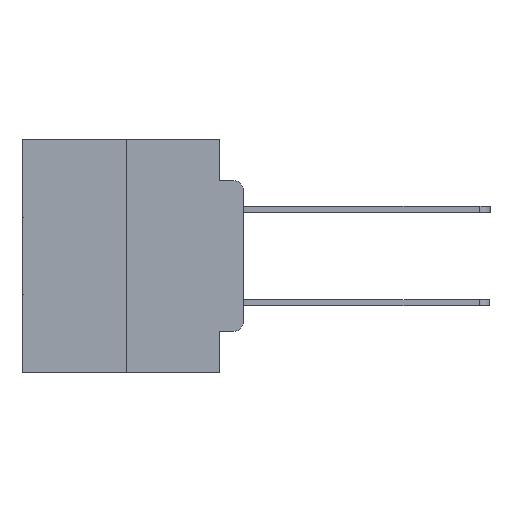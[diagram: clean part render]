
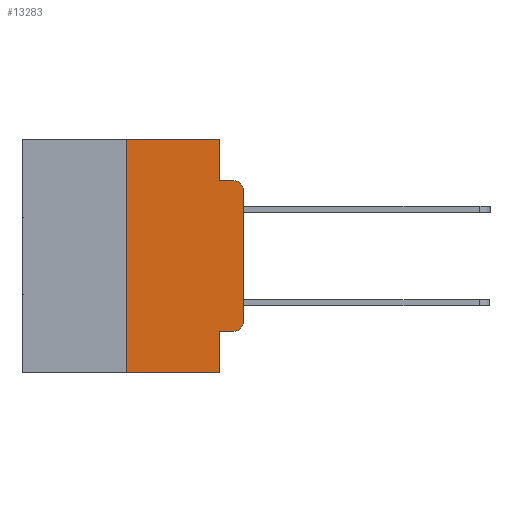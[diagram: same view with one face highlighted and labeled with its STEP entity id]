
A CAD part, left-side view. The second image highlights one B-rep face of the part: STEP entity #13283.
In plain terms, the highlighted planar face has unit normal (-1, 0, 0).
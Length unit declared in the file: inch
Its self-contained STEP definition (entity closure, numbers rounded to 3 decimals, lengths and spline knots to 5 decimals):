
#74 = LINE ( 'NONE', #17352, #17470 ) ;
#259 = EDGE_CURVE ( 'NONE', #20499, #8389, #25145, .T. ) ;
#505 = AXIS2_PLACEMENT_3D ( 'NONE', #17555, #4078, #19774 ) ;
#2021 = LINE ( 'NONE', #19113, #19306 ) ;
#2172 = CARTESIAN_POINT ( 'NONE',  ( 0., 0.051, 0. ) ) ;
#2470 = CARTESIAN_POINT ( 'NONE',  ( 0., 0.02, -0.1085 ) ) ;
#2511 = CIRCLE ( 'NONE', #24557, 0.02 ) ;
#2782 = VECTOR ( 'NONE', #16521, 39.37008 ) ;
#2895 = DIRECTION ( 'NONE',  ( 0., -1., 0. ) ) ;
#3083 = DIRECTION ( 'NONE',  ( 0., -1., 0. ) ) ;
#3151 = EDGE_CURVE ( 'NONE', #23334, #11149, #12526, .T. ) ;
#3281 = DIRECTION ( 'NONE',  ( 0., 0., -1. ) ) ;
#3370 = DIRECTION ( 'NONE',  ( -1., 0., 0. ) ) ;
#3876 = ORIENTED_EDGE ( 'NONE', *, *, #259, .T. ) ;
#3967 = ORIENTED_EDGE ( 'NONE', *, *, #23420, .T. ) ;
#4000 = EDGE_CURVE ( 'NONE', #27814, #16718, #27619, .T. ) ;
#4019 = VECTOR ( 'NONE', #2895, 39.37008 ) ;
#4078 = DIRECTION ( 'NONE',  ( 1., 0., 0. ) ) ;
#4799 = DIRECTION ( 'NONE',  ( 0., 0., -1. ) ) ;
#5612 = CARTESIAN_POINT ( 'NONE',  ( 0., 0.051, -0.0885 ) ) ;
#6364 = VERTEX_POINT ( 'NONE', #13556 ) ;
#7198 = ORIENTED_EDGE ( 'NONE', *, *, #21034, .F. ) ;
#7343 = ORIENTED_EDGE ( 'NONE', *, *, #3151, .F. ) ;
#8389 = VERTEX_POINT ( 'NONE', #17663 ) ;
#8488 = ORIENTED_EDGE ( 'NONE', *, *, #8884, .F. ) ;
#8609 = CARTESIAN_POINT ( 'NONE',  ( 0., 0.25, 0. ) ) ;
#8785 = ORIENTED_EDGE ( 'NONE', *, *, #18581, .F. ) ;
#8884 = EDGE_CURVE ( 'NONE', #16817, #23334, #74, .T. ) ;
#9549 = ORIENTED_EDGE ( 'NONE', *, *, #4000, .T. ) ;
#10341 = ORIENTED_EDGE ( 'NONE', *, *, #25168, .F. ) ;
#10415 = ORIENTED_EDGE ( 'NONE', *, *, #19322, .T. ) ;
#11014 = ORIENTED_EDGE ( 'NONE', *, *, #17823, .T. ) ;
#11149 = VERTEX_POINT ( 'NONE', #5612 ) ;
#11179 = CARTESIAN_POINT ( 'NONE',  ( 0., 0.02, -0.0885 ) ) ;
#11889 = CARTESIAN_POINT ( 'NONE',  ( 0., 0.473, -0.5 ) ) ;
#12076 = CARTESIAN_POINT ( 'NONE',  ( 0., 0., 0. ) ) ;
#12526 = LINE ( 'NONE', #16990, #24297 ) ;
#12701 = CARTESIAN_POINT ( 'NONE',  ( 0., 0.051, -0.5 ) ) ;
#13260 = LINE ( 'NONE', #18723, #24316 ) ;
#13283 = ADVANCED_FACE ( 'NONE', ( #22007 ), #24064, .F. ) ;
#13556 = CARTESIAN_POINT ( 'NONE',  ( 0., 0.051, -0.4115 ) ) ;
#14378 = CARTESIAN_POINT ( 'NONE',  ( 0., 0.25, 0. ) ) ;
#15925 = DIRECTION ( 'NONE',  ( 0., 0., -1. ) ) ;
#16521 = DIRECTION ( 'NONE',  ( 0., 0., 1. ) ) ;
#16628 = DIRECTION ( 'NONE',  ( 0., 0., 1. ) ) ;
#16718 = VERTEX_POINT ( 'NONE', #12701 ) ;
#16817 = VERTEX_POINT ( 'NONE', #8609 ) ;
#16868 = CARTESIAN_POINT ( 'NONE',  ( 0., 0.02, -0.3915 ) ) ;
#16990 = CARTESIAN_POINT ( 'NONE',  ( 0., 0.051, 0. ) ) ;
#17352 = CARTESIAN_POINT ( 'NONE',  ( 0., 0.473, 0. ) ) ;
#17470 = VECTOR ( 'NONE', #19581, 39.37008 ) ;
#17555 = CARTESIAN_POINT ( 'NONE',  ( 0., 0.473, 0. ) ) ;
#17663 = CARTESIAN_POINT ( 'NONE',  ( 0., 0., -0.1085 ) ) ;
#17823 = EDGE_CURVE ( 'NONE', #27880, #20499, #23506, .T. ) ;
#18232 = DIRECTION ( 'NONE',  ( -1., 0., 0. ) ) ;
#18581 = EDGE_CURVE ( 'NONE', #27814, #16817, #26158, .T. ) ;
#18723 = CARTESIAN_POINT ( 'NONE',  ( 0., 0.051, -0.0885 ) ) ;
#19090 = DIRECTION ( 'NONE',  ( 0., 0., -1. ) ) ;
#19113 = CARTESIAN_POINT ( 'NONE',  ( 0., 0.051, -0.4115 ) ) ;
#19306 = VECTOR ( 'NONE', #21339, 39.37008 ) ;
#19322 = EDGE_CURVE ( 'NONE', #6364, #27880, #2021, .T. ) ;
#19581 = DIRECTION ( 'NONE',  ( 0., -1., 0. ) ) ;
#19774 = DIRECTION ( 'NONE',  ( 0., 0., -1. ) ) ;
#20499 = VERTEX_POINT ( 'NONE', #20874 ) ;
#20874 = CARTESIAN_POINT ( 'NONE',  ( 0., 0., -0.3915 ) ) ;
#21034 = EDGE_CURVE ( 'NONE', #11149, #27035, #13260, .T. ) ;
#21067 = VECTOR ( 'NONE', #16628, 39.37008 ) ;
#21339 = DIRECTION ( 'NONE',  ( 0., -1., 0. ) ) ;
#22007 = FACE_OUTER_BOUND ( 'NONE', #27049, .T. ) ;
#23334 = VERTEX_POINT ( 'NONE', #2172 ) ;
#23420 = EDGE_CURVE ( 'NONE', #8389, #27035, #2511, .T. ) ;
#23506 = CIRCLE ( 'NONE', #27523, 0.02 ) ;
#24064 = PLANE ( 'NONE',  #505 ) ;
#24297 = VECTOR ( 'NONE', #3281, 39.37008 ) ;
#24316 = VECTOR ( 'NONE', #3083, 39.37008 ) ;
#24557 = AXIS2_PLACEMENT_3D ( 'NONE', #2470, #18232, #4799 ) ;
#25145 = LINE ( 'NONE', #12076, #2782 ) ;
#25168 = EDGE_CURVE ( 'NONE', #6364, #16718, #28742, .T. ) ;
#25715 = CARTESIAN_POINT ( 'NONE',  ( 0., 0.02, -0.4115 ) ) ;
#26158 = LINE ( 'NONE', #14378, #21067 ) ;
#26841 = CARTESIAN_POINT ( 'NONE',  ( 0., 0.051, 0. ) ) ;
#27035 = VERTEX_POINT ( 'NONE', #11179 ) ;
#27049 = EDGE_LOOP ( 'NONE', ( #3876, #3967, #7198, #7343, #8488, #8785, #9549, #10341, #10415, #11014 ) ) ;
#27523 = AXIS2_PLACEMENT_3D ( 'NONE', #16868, #3370, #19090 ) ;
#27619 = LINE ( 'NONE', #11889, #4019 ) ;
#27683 = CARTESIAN_POINT ( 'NONE',  ( 0., 0.25, -0.5 ) ) ;
#27814 = VERTEX_POINT ( 'NONE', #27683 ) ;
#27880 = VERTEX_POINT ( 'NONE', #25715 ) ;
#28086 = VECTOR ( 'NONE', #15925, 39.37008 ) ;
#28742 = LINE ( 'NONE', #26841, #28086 ) ;
